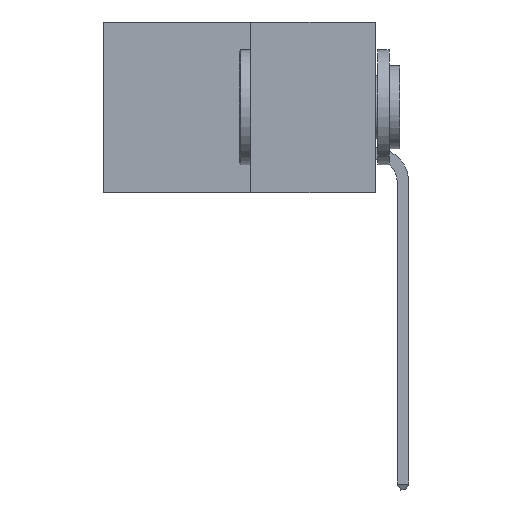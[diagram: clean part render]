
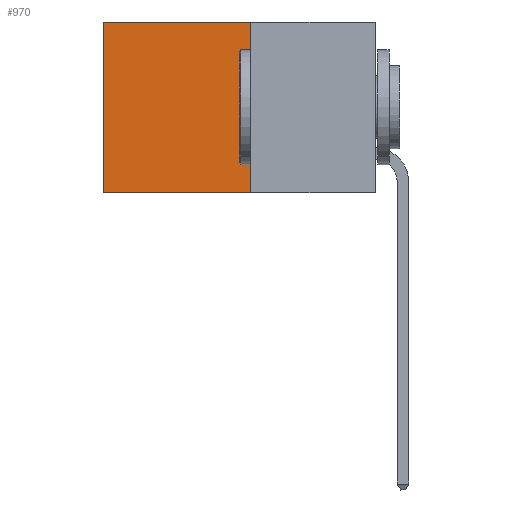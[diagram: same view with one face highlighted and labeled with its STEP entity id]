
A CAD part, left-side view. The second image highlights one B-rep face of the part: STEP entity #970.
In plain terms, the highlighted planar face has unit normal (-1, 0, 0).
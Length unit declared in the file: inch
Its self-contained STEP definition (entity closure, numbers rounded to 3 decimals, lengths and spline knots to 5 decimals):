
#34 = CARTESIAN_POINT ( 'NONE',  ( 0.277, 0.27, -0.37 ) ) ;
#60 = EDGE_CURVE ( 'NONE', #4580, #7238, #8109, .T. ) ;
#355 = EDGE_LOOP ( 'NONE', ( #1915, #7001, #1856, #6666 ) ) ;
#458 = PLANE ( 'NONE',  #770 ) ;
#511 = DIRECTION ( 'NONE',  ( 0., 1., 0. ) ) ;
#602 = CARTESIAN_POINT ( 'NONE',  ( 0.277, 0.27, 0. ) ) ;
#770 = AXIS2_PLACEMENT_3D ( 'NONE', #2623, #7573, #3319 ) ;
#970 = ADVANCED_FACE ( 'NONE', ( #1013 ), #458, .F. ) ;
#1013 = FACE_OUTER_BOUND ( 'NONE', #355, .T. ) ;
#1856 = ORIENTED_EDGE ( 'NONE', *, *, #60, .F. ) ;
#1915 = ORIENTED_EDGE ( 'NONE', *, *, #3610, .T. ) ;
#2497 = DIRECTION ( 'NONE',  ( 0., 0., -1. ) ) ;
#2509 = LINE ( 'NONE', #5501, #6280 ) ;
#2623 = CARTESIAN_POINT ( 'NONE',  ( 0.277, 0.27, -0.37 ) ) ;
#2828 = CARTESIAN_POINT ( 'NONE',  ( 0.277, 0.59, 0. ) ) ;
#3097 = VECTOR ( 'NONE', #2497, 39.37008 ) ;
#3318 = EDGE_CURVE ( 'NONE', #4580, #5359, #8732, .T. ) ;
#3319 = DIRECTION ( 'NONE',  ( 0., 0., -1. ) ) ;
#3610 = EDGE_CURVE ( 'NONE', #5359, #9221, #2509, .T. ) ;
#4074 = DIRECTION ( 'NONE',  ( 0., 0., -1. ) ) ;
#4580 = VERTEX_POINT ( 'NONE', #602 ) ;
#4763 = CARTESIAN_POINT ( 'NONE',  ( 0.277, 0.27, -0.37 ) ) ;
#5359 = VERTEX_POINT ( 'NONE', #2828 ) ;
#5501 = CARTESIAN_POINT ( 'NONE',  ( 0.277, 0.59, -0.37 ) ) ;
#6131 = EDGE_CURVE ( 'NONE', #7238, #9221, #6724, .T. ) ;
#6280 = VECTOR ( 'NONE', #4074, 39.37008 ) ;
#6498 = VECTOR ( 'NONE', #6893, 39.37008 ) ;
#6606 = VECTOR ( 'NONE', #511, 39.37008 ) ;
#6666 = ORIENTED_EDGE ( 'NONE', *, *, #3318, .T. ) ;
#6724 = LINE ( 'NONE', #4763, #6498 ) ;
#6893 = DIRECTION ( 'NONE',  ( 0., 1., 0. ) ) ;
#7001 = ORIENTED_EDGE ( 'NONE', *, *, #6131, .F. ) ;
#7238 = VERTEX_POINT ( 'NONE', #34 ) ;
#7573 = DIRECTION ( 'NONE',  ( 1., 0., 0. ) ) ;
#8107 = CARTESIAN_POINT ( 'NONE',  ( 0.277, 0.59, -0.37 ) ) ;
#8109 = LINE ( 'NONE', #8957, #3097 ) ;
#8336 = CARTESIAN_POINT ( 'NONE',  ( 0.277, 0.27, 0. ) ) ;
#8732 = LINE ( 'NONE', #8336, #6606 ) ;
#8957 = CARTESIAN_POINT ( 'NONE',  ( 0.277, 0.27, -0.37 ) ) ;
#9221 = VERTEX_POINT ( 'NONE', #8107 ) ;
